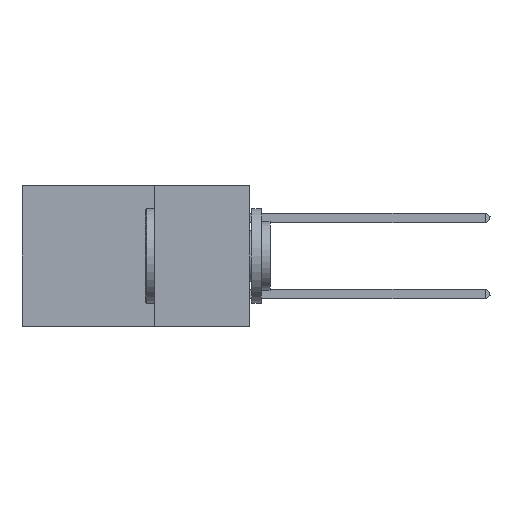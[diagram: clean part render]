
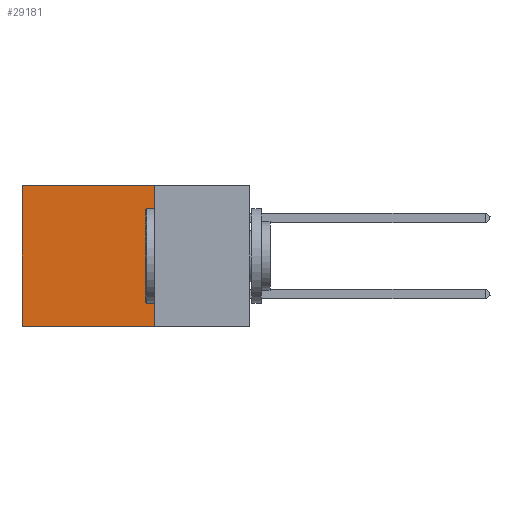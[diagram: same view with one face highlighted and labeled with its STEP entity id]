
A CAD part, left-side view. The second image highlights one B-rep face of the part: STEP entity #29181.
In plain terms, the highlighted planar face has unit normal (-1, 0, 0).
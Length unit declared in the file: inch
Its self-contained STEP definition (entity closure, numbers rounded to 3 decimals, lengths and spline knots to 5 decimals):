
#1099 = EDGE_CURVE ( 'NONE', #22790, #41385, #42837, .T. ) ;
#1732 = LINE ( 'NONE', #2386, #34329 ) ;
#2386 = CARTESIAN_POINT ( 'NONE',  ( 0.2875, 0.25, -0.37 ) ) ;
#4377 = DIRECTION ( 'NONE',  ( 1., 0., 0. ) ) ;
#5420 = CARTESIAN_POINT ( 'NONE',  ( 0.2875, 0.6, 0. ) ) ;
#6303 = LINE ( 'NONE', #26217, #14867 ) ;
#7536 = VERTEX_POINT ( 'NONE', #26291 ) ;
#8593 = EDGE_LOOP ( 'NONE', ( #19239, #46829, #40323, #33122 ) ) ;
#9394 = EDGE_CURVE ( 'NONE', #34898, #7536, #1732, .T. ) ;
#14867 = VECTOR ( 'NONE', #25915, 39.37008 ) ;
#15238 = PLANE ( 'NONE',  #17524 ) ;
#17524 = AXIS2_PLACEMENT_3D ( 'NONE', #26236, #4377, #33745 ) ;
#19239 = ORIENTED_EDGE ( 'NONE', *, *, #20055, .T. ) ;
#20055 = EDGE_CURVE ( 'NONE', #41385, #7536, #32055, .T. ) ;
#22673 = CARTESIAN_POINT ( 'NONE',  ( 0.2875, 0.25, 0. ) ) ;
#22790 = VERTEX_POINT ( 'NONE', #43654 ) ;
#25915 = DIRECTION ( 'NONE',  ( 0., 0., -1. ) ) ;
#26217 = CARTESIAN_POINT ( 'NONE',  ( 0.2875, 0.25, 0. ) ) ;
#26236 = CARTESIAN_POINT ( 'NONE',  ( 0.2875, 0.25, 0. ) ) ;
#26291 = CARTESIAN_POINT ( 'NONE',  ( 0.2875, 0.6, -0.37 ) ) ;
#27762 = DIRECTION ( 'NONE',  ( 0., 1., 0. ) ) ;
#28967 = CARTESIAN_POINT ( 'NONE',  ( 0.2875, 0.25, -0.37 ) ) ;
#29181 = ADVANCED_FACE ( 'NONE', ( #37848 ), #15238, .F. ) ;
#29837 = DIRECTION ( 'NONE',  ( 0., 1., 0. ) ) ;
#30951 = DIRECTION ( 'NONE',  ( 0., 0., -1. ) ) ;
#32055 = LINE ( 'NONE', #5420, #38304 ) ;
#32607 = VECTOR ( 'NONE', #29837, 39.37008 ) ;
#33122 = ORIENTED_EDGE ( 'NONE', *, *, #1099, .T. ) ;
#33745 = DIRECTION ( 'NONE',  ( 0., 0., -1. ) ) ;
#34329 = VECTOR ( 'NONE', #27762, 39.37008 ) ;
#34898 = VERTEX_POINT ( 'NONE', #28967 ) ;
#37339 = CARTESIAN_POINT ( 'NONE',  ( 0.2875, 0.6, 0. ) ) ;
#37848 = FACE_OUTER_BOUND ( 'NONE', #8593, .T. ) ;
#38304 = VECTOR ( 'NONE', #30951, 39.37008 ) ;
#40323 = ORIENTED_EDGE ( 'NONE', *, *, #45759, .F. ) ;
#41385 = VERTEX_POINT ( 'NONE', #37339 ) ;
#42837 = LINE ( 'NONE', #22673, #32607 ) ;
#43654 = CARTESIAN_POINT ( 'NONE',  ( 0.2875, 0.25, 0. ) ) ;
#45759 = EDGE_CURVE ( 'NONE', #22790, #34898, #6303, .T. ) ;
#46829 = ORIENTED_EDGE ( 'NONE', *, *, #9394, .F. ) ;
